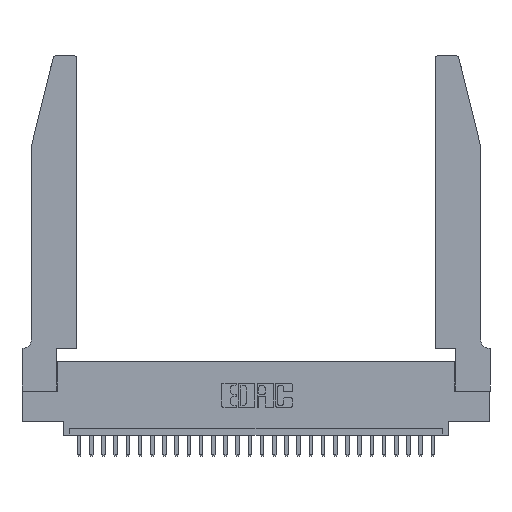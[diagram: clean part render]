
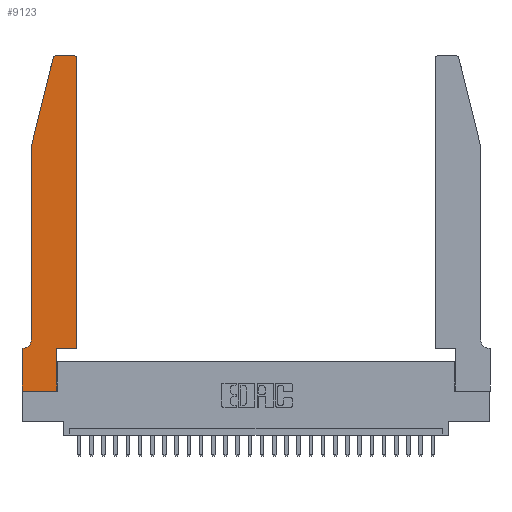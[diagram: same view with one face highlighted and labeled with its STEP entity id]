
A CAD part, top view. The second image highlights one B-rep face of the part: STEP entity #9123.
In plain terms, the highlighted planar face has unit normal (0, 0, 1).
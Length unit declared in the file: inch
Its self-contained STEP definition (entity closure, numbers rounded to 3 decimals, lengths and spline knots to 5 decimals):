
#346 = DIRECTION ( 'NONE',  ( 1., 0., 0. ) ) ;
#373 = AXIS2_PLACEMENT_3D ( 'NONE', #5454, #21196, #12045 ) ;
#600 = CARTESIAN_POINT ( 'NONE',  ( 0.4205, 2.75, 0.37 ) ) ;
#1155 = DIRECTION ( 'NONE',  ( 0., 1., 0. ) ) ;
#1777 = DIRECTION ( 'NONE',  ( 0., 0., 1. ) ) ;
#1833 = CARTESIAN_POINT ( 'NONE',  ( 0.4505, 2.72, 0.37 ) ) ;
#1894 = EDGE_CURVE ( 'NONE', #27358, #27923, #24354, .T. ) ;
#2413 = VERTEX_POINT ( 'NONE', #15365 ) ;
#2891 = VECTOR ( 'NONE', #1155, 39.37008 ) ;
#2918 = VECTOR ( 'NONE', #14866, 39.37008 ) ;
#3443 = VECTOR ( 'NONE', #4281, 39.37008 ) ;
#3525 = CIRCLE ( 'NONE', #26215, 0.03 ) ;
#3796 = CARTESIAN_POINT ( 'NONE',  ( 0.2865, 0.35, 0.37 ) ) ;
#3816 = CARTESIAN_POINT ( 'NONE',  ( 0., 0.35, 0.37 ) ) ;
#4083 = LINE ( 'NONE', #13799, #25246 ) ;
#4145 = EDGE_CURVE ( 'NONE', #5981, #2413, #10094, .T. ) ;
#4281 = DIRECTION ( 'NONE',  ( -1., 0., 0. ) ) ;
#4830 = DIRECTION ( 'NONE',  ( 0., 0., -1. ) ) ;
#5454 = CARTESIAN_POINT ( 'NONE',  ( 0.284, 2.72, 0.37 ) ) ;
#5555 = ORIENTED_EDGE ( 'NONE', *, *, #1894, .T. ) ;
#5638 = VERTEX_POINT ( 'NONE', #10656 ) ;
#5687 = CARTESIAN_POINT ( 'NONE',  ( 0.4505, 0.35, 0.37 ) ) ;
#5978 = LINE ( 'NONE', #11699, #7409 ) ;
#5981 = VERTEX_POINT ( 'NONE', #14001 ) ;
#6060 = CARTESIAN_POINT ( 'NONE',  ( 0., 0., 0.37 ) ) ;
#6407 = EDGE_CURVE ( 'NONE', #23375, #5981, #21645, .T. ) ;
#6887 = VECTOR ( 'NONE', #23830, 39.37008 ) ;
#7036 = DIRECTION ( 'NONE',  ( 0., 1., 0. ) ) ;
#7409 = VECTOR ( 'NONE', #20755, 39.37008 ) ;
#7510 = ORIENTED_EDGE ( 'NONE', *, *, #12352, .T. ) ;
#7859 = EDGE_CURVE ( 'NONE', #8317, #13793, #3525, .T. ) ;
#8317 = VERTEX_POINT ( 'NONE', #1833 ) ;
#8515 = CARTESIAN_POINT ( 'NONE',  ( 0., 0., 0.37 ) ) ;
#8699 = EDGE_CURVE ( 'NONE', #13793, #8889, #10180, .T. ) ;
#8889 = VERTEX_POINT ( 'NONE', #10302 ) ;
#9010 = CARTESIAN_POINT ( 'NONE',  ( 0.0755, 2., 0.37 ) ) ;
#9123 = ADVANCED_FACE ( 'NONE', ( #20381 ), #19858, .T. ) ;
#9883 = EDGE_CURVE ( 'NONE', #27923, #19853, #18590, .T. ) ;
#10094 = CIRCLE ( 'NONE', #15425, 0.07 ) ;
#10180 = LINE ( 'NONE', #20203, #3443 ) ;
#10302 = CARTESIAN_POINT ( 'NONE',  ( 0.284, 2.75, 0.37 ) ) ;
#10576 = AXIS2_PLACEMENT_3D ( 'NONE', #3816, #1777, #24260 ) ;
#10656 = CARTESIAN_POINT ( 'NONE',  ( 0., 0.35, 0.37 ) ) ;
#11338 = VECTOR ( 'NONE', #20429, 39.37008 ) ;
#11421 = EDGE_CURVE ( 'NONE', #8889, #12981, #17114, .T. ) ;
#11699 = CARTESIAN_POINT ( 'NONE',  ( 0.0755, 0.35, 0.37 ) ) ;
#11791 = CARTESIAN_POINT ( 'NONE',  ( 0.0055, 0.42, 0.37 ) ) ;
#11873 = ORIENTED_EDGE ( 'NONE', *, *, #11421, .T. ) ;
#12045 = DIRECTION ( 'NONE',  ( 1., 0., 0. ) ) ;
#12352 = EDGE_CURVE ( 'NONE', #25304, #8317, #18458, .T. ) ;
#12981 = VERTEX_POINT ( 'NONE', #18047 ) ;
#13793 = VERTEX_POINT ( 'NONE', #600 ) ;
#13799 = CARTESIAN_POINT ( 'NONE',  ( 0.4505, 0.35, 0.37 ) ) ;
#14001 = CARTESIAN_POINT ( 'NONE',  ( 0.0755, 0.42, 0.37 ) ) ;
#14020 = VECTOR ( 'NONE', #7036, 39.37008 ) ;
#14610 = CARTESIAN_POINT ( 'NONE',  ( 0.2865, 0., 0.37 ) ) ;
#14866 = DIRECTION ( 'NONE',  ( 0., -1., 0. ) ) ;
#15365 = CARTESIAN_POINT ( 'NONE',  ( 0.0055, 0.35, 0.37 ) ) ;
#15425 = AXIS2_PLACEMENT_3D ( 'NONE', #11791, #4830, #27909 ) ;
#16134 = ORIENTED_EDGE ( 'NONE', *, *, #4145, .T. ) ;
#16189 = CARTESIAN_POINT ( 'NONE',  ( 0., 0., 0.37 ) ) ;
#16604 = EDGE_CURVE ( 'NONE', #2413, #5638, #5978, .T. ) ;
#16615 = CARTESIAN_POINT ( 'NONE',  ( 0.0755, 2., 0.37 ) ) ;
#16904 = VECTOR ( 'NONE', #26860, 39.37008 ) ;
#17114 = CIRCLE ( 'NONE', #373, 0.03 ) ;
#18047 = CARTESIAN_POINT ( 'NONE',  ( 0.25487, 2.72718, 0.37 ) ) ;
#18458 = LINE ( 'NONE', #5687, #2891 ) ;
#18529 = ORIENTED_EDGE ( 'NONE', *, *, #21447, .T. ) ;
#18571 = EDGE_CURVE ( 'NONE', #19853, #25304, #4083, .T. ) ;
#18590 = LINE ( 'NONE', #21835, #14020 ) ;
#18681 = LINE ( 'NONE', #26679, #16904 ) ;
#18770 = ORIENTED_EDGE ( 'NONE', *, *, #26107, .T. ) ;
#19853 = VERTEX_POINT ( 'NONE', #3796 ) ;
#19858 = PLANE ( 'NONE',  #10576 ) ;
#20203 = CARTESIAN_POINT ( 'NONE',  ( 0.2605, 2.75, 0.37 ) ) ;
#20381 = FACE_OUTER_BOUND ( 'NONE', #21889, .T. ) ;
#20429 = DIRECTION ( 'NONE',  ( 1., 0., 0. ) ) ;
#20755 = DIRECTION ( 'NONE',  ( -1., 0., 0. ) ) ;
#21196 = DIRECTION ( 'NONE',  ( 0., 0., 1. ) ) ;
#21357 = ORIENTED_EDGE ( 'NONE', *, *, #6407, .T. ) ;
#21447 = EDGE_CURVE ( 'NONE', #5638, #27358, #25932, .T. ) ;
#21645 = LINE ( 'NONE', #9010, #2918 ) ;
#21700 = ORIENTED_EDGE ( 'NONE', *, *, #8699, .T. ) ;
#21835 = CARTESIAN_POINT ( 'NONE',  ( 0.2865, 0.35, 0.37 ) ) ;
#21889 = EDGE_LOOP ( 'NONE', ( #21700, #11873, #18770, #21357, #16134, #23464, #18529, #5555, #25068, #22545, #7510, #25101 ) ) ;
#22545 = ORIENTED_EDGE ( 'NONE', *, *, #18571, .T. ) ;
#23375 = VERTEX_POINT ( 'NONE', #16615 ) ;
#23464 = ORIENTED_EDGE ( 'NONE', *, *, #16604, .T. ) ;
#23784 = CARTESIAN_POINT ( 'NONE',  ( 0.4505, 0.35, 0.37 ) ) ;
#23830 = DIRECTION ( 'NONE',  ( 0., -1., 0. ) ) ;
#24260 = DIRECTION ( 'NONE',  ( 1., 0., 0. ) ) ;
#24354 = LINE ( 'NONE', #16189, #11338 ) ;
#25068 = ORIENTED_EDGE ( 'NONE', *, *, #9883, .T. ) ;
#25101 = ORIENTED_EDGE ( 'NONE', *, *, #7859, .T. ) ;
#25246 = VECTOR ( 'NONE', #346, 39.37008 ) ;
#25304 = VERTEX_POINT ( 'NONE', #23784 ) ;
#25932 = LINE ( 'NONE', #6060, #6887 ) ;
#26107 = EDGE_CURVE ( 'NONE', #12981, #23375, #18681, .T. ) ;
#26215 = AXIS2_PLACEMENT_3D ( 'NONE', #28755, #26276, #28550 ) ;
#26276 = DIRECTION ( 'NONE',  ( 0., 0., 1. ) ) ;
#26679 = CARTESIAN_POINT ( 'NONE',  ( 0.0755, 2., 0.37 ) ) ;
#26860 = DIRECTION ( 'NONE',  ( -0.239, -0.971, 0. ) ) ;
#27358 = VERTEX_POINT ( 'NONE', #8515 ) ;
#27909 = DIRECTION ( 'NONE',  ( -1., 0., 0. ) ) ;
#27923 = VERTEX_POINT ( 'NONE', #14610 ) ;
#28550 = DIRECTION ( 'NONE',  ( 1., 0., 0. ) ) ;
#28755 = CARTESIAN_POINT ( 'NONE',  ( 0.4205, 2.72, 0.37 ) ) ;
